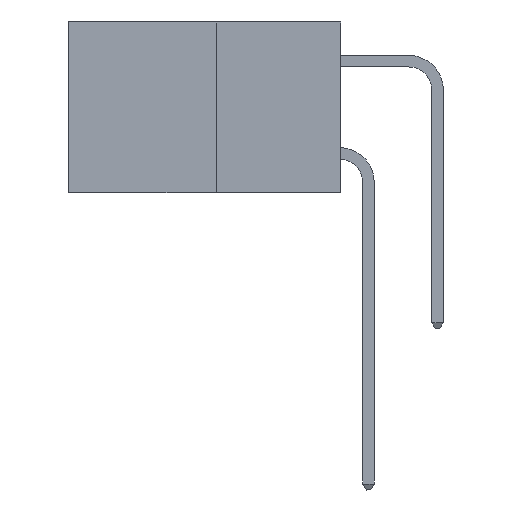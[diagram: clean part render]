
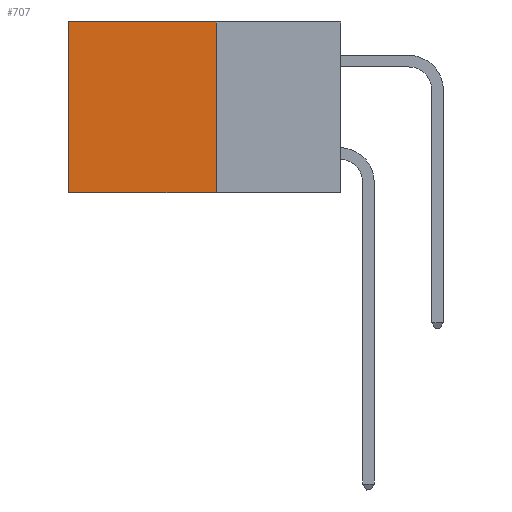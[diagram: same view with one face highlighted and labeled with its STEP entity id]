
A CAD part, left-side view. The second image highlights one B-rep face of the part: STEP entity #707.
In plain terms, the highlighted planar face has unit normal (-1, 0, 0).
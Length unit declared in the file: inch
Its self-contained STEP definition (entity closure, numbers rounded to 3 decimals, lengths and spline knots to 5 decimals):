
#447 = CARTESIAN_POINT ( 'NONE',  ( 0.277, 0.27, -0.37 ) ) ;
#670 = VERTEX_POINT ( 'NONE', #6005 ) ;
#707 = ADVANCED_FACE ( 'NONE', ( #1335 ), #7230, .F. ) ;
#1335 = FACE_OUTER_BOUND ( 'NONE', #5395, .T. ) ;
#2210 = ORIENTED_EDGE ( 'NONE', *, *, #8501, .F. ) ;
#2213 = DIRECTION ( 'NONE',  ( 0., 0., -1. ) ) ;
#2221 = VECTOR ( 'NONE', #6030, 39.37008 ) ;
#2240 = CARTESIAN_POINT ( 'NONE',  ( 0.277, 0.59, -0.37 ) ) ;
#2271 = AXIS2_PLACEMENT_3D ( 'NONE', #7693, #6451, #8907 ) ;
#2798 = LINE ( 'NONE', #2240, #8613 ) ;
#3769 = CARTESIAN_POINT ( 'NONE',  ( 0.277, 0.27, 0. ) ) ;
#4005 = ORIENTED_EDGE ( 'NONE', *, *, #7921, .T. ) ;
#4112 = VERTEX_POINT ( 'NONE', #5920 ) ;
#4260 = ORIENTED_EDGE ( 'NONE', *, *, #7251, .T. ) ;
#4265 = LINE ( 'NONE', #6154, #2221 ) ;
#4466 = DIRECTION ( 'NONE',  ( 0., 1., 0. ) ) ;
#4496 = VERTEX_POINT ( 'NONE', #3769 ) ;
#4754 = CARTESIAN_POINT ( 'NONE',  ( 0.277, 0.27, -0.37 ) ) ;
#5058 = CARTESIAN_POINT ( 'NONE',  ( 0.277, 0.59, 0. ) ) ;
#5395 = EDGE_LOOP ( 'NONE', ( #4005, #6050, #2210, #4260 ) ) ;
#5533 = DIRECTION ( 'NONE',  ( 0., 0., -1. ) ) ;
#5828 = LINE ( 'NONE', #447, #7342 ) ;
#5920 = CARTESIAN_POINT ( 'NONE',  ( 0.277, 0.27, -0.37 ) ) ;
#6005 = CARTESIAN_POINT ( 'NONE',  ( 0.277, 0.59, -0.37 ) ) ;
#6030 = DIRECTION ( 'NONE',  ( 0., 1., 0. ) ) ;
#6050 = ORIENTED_EDGE ( 'NONE', *, *, #9724, .F. ) ;
#6154 = CARTESIAN_POINT ( 'NONE',  ( 0.277, 0.27, 0. ) ) ;
#6451 = DIRECTION ( 'NONE',  ( 1., 0., 0. ) ) ;
#7230 = PLANE ( 'NONE',  #2271 ) ;
#7251 = EDGE_CURVE ( 'NONE', #4496, #9567, #4265, .T. ) ;
#7342 = VECTOR ( 'NONE', #4466, 39.37008 ) ;
#7693 = CARTESIAN_POINT ( 'NONE',  ( 0.277, 0.27, -0.37 ) ) ;
#7921 = EDGE_CURVE ( 'NONE', #9567, #670, #2798, .T. ) ;
#8501 = EDGE_CURVE ( 'NONE', #4496, #4112, #9219, .T. ) ;
#8613 = VECTOR ( 'NONE', #2213, 39.37008 ) ;
#8907 = DIRECTION ( 'NONE',  ( 0., 0., -1. ) ) ;
#8977 = VECTOR ( 'NONE', #5533, 39.37008 ) ;
#9219 = LINE ( 'NONE', #4754, #8977 ) ;
#9567 = VERTEX_POINT ( 'NONE', #5058 ) ;
#9724 = EDGE_CURVE ( 'NONE', #4112, #670, #5828, .T. ) ;
